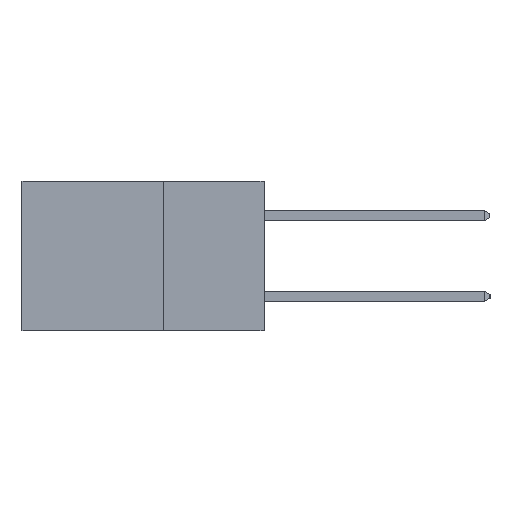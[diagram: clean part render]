
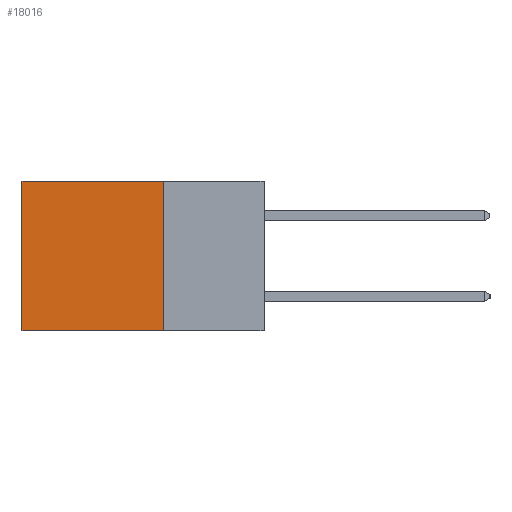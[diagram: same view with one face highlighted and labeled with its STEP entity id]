
A CAD part, left-side view. The second image highlights one B-rep face of the part: STEP entity #18016.
In plain terms, the highlighted planar face has unit normal (-1, 0, 0).
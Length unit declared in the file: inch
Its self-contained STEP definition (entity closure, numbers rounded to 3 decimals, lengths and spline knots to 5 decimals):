
#29 = VECTOR ( 'NONE', #262, 39.37008 ) ;
#262 = DIRECTION ( 'NONE',  ( 0., 1., 0. ) ) ;
#471 = DIRECTION ( 'NONE',  ( 0., 0., -1. ) ) ;
#1470 = EDGE_LOOP ( 'NONE', ( #21859, #24531, #23783, #7370 ) ) ;
#1505 = CARTESIAN_POINT ( 'NONE',  ( 0.2615, 0.6, 0. ) ) ;
#2325 = DIRECTION ( 'NONE',  ( 0., 0., -1. ) ) ;
#5222 = LINE ( 'NONE', #8019, #29 ) ;
#5488 = PLANE ( 'NONE',  #9330 ) ;
#7011 = VERTEX_POINT ( 'NONE', #14069 ) ;
#7155 = LINE ( 'NONE', #8043, #22080 ) ;
#7370 = ORIENTED_EDGE ( 'NONE', *, *, #16261, .T. ) ;
#7657 = CARTESIAN_POINT ( 'NONE',  ( 0.2615, 0.25, 0. ) ) ;
#8019 = CARTESIAN_POINT ( 'NONE',  ( 0.2615, 0.25, 0. ) ) ;
#8043 = CARTESIAN_POINT ( 'NONE',  ( 0.2615, 0.25, -0.37 ) ) ;
#9330 = AXIS2_PLACEMENT_3D ( 'NONE', #23049, #11438, #25004 ) ;
#9996 = DIRECTION ( 'NONE',  ( 0., 1., 0. ) ) ;
#10068 = CARTESIAN_POINT ( 'NONE',  ( 0.2615, 0.6, -0.37 ) ) ;
#11085 = EDGE_CURVE ( 'NONE', #7011, #15327, #7155, .T. ) ;
#11438 = DIRECTION ( 'NONE',  ( 1., 0., 0. ) ) ;
#11930 = EDGE_CURVE ( 'NONE', #14826, #15327, #18070, .T. ) ;
#12909 = VECTOR ( 'NONE', #2325, 39.37008 ) ;
#14069 = CARTESIAN_POINT ( 'NONE',  ( 0.2615, 0.25, -0.37 ) ) ;
#14411 = VECTOR ( 'NONE', #471, 39.37008 ) ;
#14826 = VERTEX_POINT ( 'NONE', #1505 ) ;
#15327 = VERTEX_POINT ( 'NONE', #20791 ) ;
#16026 = FACE_OUTER_BOUND ( 'NONE', #1470, .T. ) ;
#16261 = EDGE_CURVE ( 'NONE', #18815, #14826, #5222, .T. ) ;
#18016 = ADVANCED_FACE ( 'NONE', ( #16026 ), #5488, .F. ) ;
#18070 = LINE ( 'NONE', #10068, #12909 ) ;
#18815 = VERTEX_POINT ( 'NONE', #7657 ) ;
#19682 = EDGE_CURVE ( 'NONE', #18815, #7011, #24703, .T. ) ;
#20791 = CARTESIAN_POINT ( 'NONE',  ( 0.2615, 0.6, -0.37 ) ) ;
#21859 = ORIENTED_EDGE ( 'NONE', *, *, #11930, .T. ) ;
#22080 = VECTOR ( 'NONE', #9996, 39.37008 ) ;
#23049 = CARTESIAN_POINT ( 'NONE',  ( 0.2615, 0.25, -0.37 ) ) ;
#23762 = CARTESIAN_POINT ( 'NONE',  ( 0.2615, 0.25, -0.37 ) ) ;
#23783 = ORIENTED_EDGE ( 'NONE', *, *, #19682, .F. ) ;
#24531 = ORIENTED_EDGE ( 'NONE', *, *, #11085, .F. ) ;
#24703 = LINE ( 'NONE', #23762, #14411 ) ;
#25004 = DIRECTION ( 'NONE',  ( 0., 0., -1. ) ) ;
